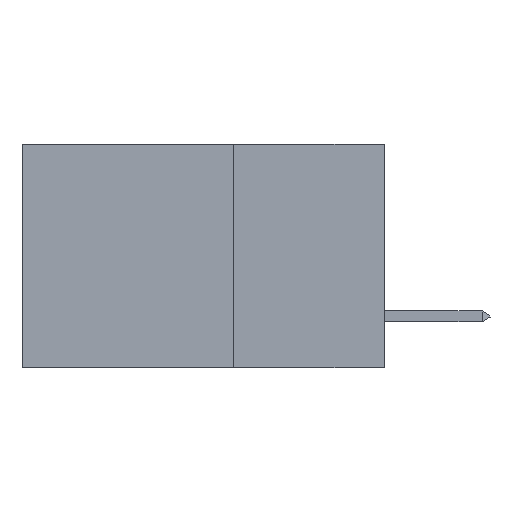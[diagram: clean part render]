
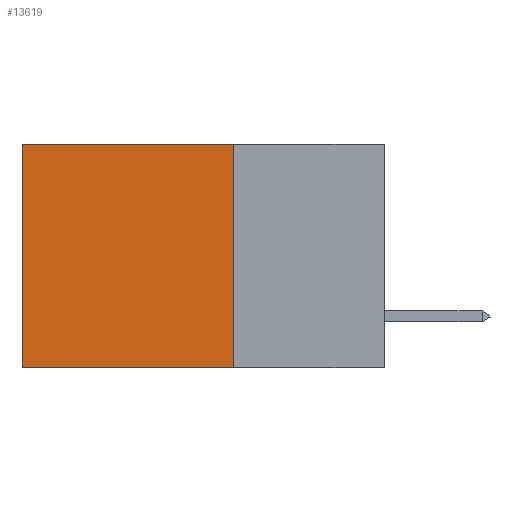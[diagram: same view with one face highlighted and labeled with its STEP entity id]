
A CAD part, left-side view. The second image highlights one B-rep face of the part: STEP entity #13619.
In plain terms, the highlighted planar face has unit normal (-1, 0, 0).
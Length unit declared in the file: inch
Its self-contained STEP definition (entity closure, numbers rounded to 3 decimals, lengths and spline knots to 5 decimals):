
#295 = EDGE_CURVE ( 'NONE', #6804, #10270, #2146, .T. ) ;
#1243 = CARTESIAN_POINT ( 'NONE',  ( 0.2875, 0.6, 0. ) ) ;
#1862 = CARTESIAN_POINT ( 'NONE',  ( 0.2875, 0.6, 0. ) ) ;
#2146 = LINE ( 'NONE', #15184, #16789 ) ;
#2931 = DIRECTION ( 'NONE',  ( 1., 0., 0. ) ) ;
#3605 = DIRECTION ( 'NONE',  ( 0., 0., -1. ) ) ;
#4009 = CARTESIAN_POINT ( 'NONE',  ( 0.2875, 0.25, 0. ) ) ;
#4480 = EDGE_CURVE ( 'NONE', #6804, #11323, #6038, .T. ) ;
#5873 = ORIENTED_EDGE ( 'NONE', *, *, #4480, .T. ) ;
#6038 = LINE ( 'NONE', #4009, #15990 ) ;
#6400 = FACE_OUTER_BOUND ( 'NONE', #13943, .T. ) ;
#6772 = ORIENTED_EDGE ( 'NONE', *, *, #13091, .T. ) ;
#6804 = VERTEX_POINT ( 'NONE', #10880 ) ;
#7690 = DIRECTION ( 'NONE',  ( 0., 1., 0. ) ) ;
#8319 = AXIS2_PLACEMENT_3D ( 'NONE', #9859, #2931, #12002 ) ;
#9859 = CARTESIAN_POINT ( 'NONE',  ( 0.2875, 0.25, 0. ) ) ;
#9945 = DIRECTION ( 'NONE',  ( 0., 1., 0. ) ) ;
#10129 = ORIENTED_EDGE ( 'NONE', *, *, #295, .F. ) ;
#10270 = VERTEX_POINT ( 'NONE', #15172 ) ;
#10651 = ORIENTED_EDGE ( 'NONE', *, *, #16809, .F. ) ;
#10689 = PLANE ( 'NONE',  #8319 ) ;
#10880 = CARTESIAN_POINT ( 'NONE',  ( 0.2875, 0.25, 0. ) ) ;
#11086 = CARTESIAN_POINT ( 'NONE',  ( 0.2875, 0.6, -0.37 ) ) ;
#11323 = VERTEX_POINT ( 'NONE', #1862 ) ;
#12002 = DIRECTION ( 'NONE',  ( 0., 0., -1. ) ) ;
#12082 = LINE ( 'NONE', #16307, #13721 ) ;
#12824 = DIRECTION ( 'NONE',  ( 0., 0., -1. ) ) ;
#13091 = EDGE_CURVE ( 'NONE', #11323, #14695, #14935, .T. ) ;
#13619 = ADVANCED_FACE ( 'NONE', ( #6400 ), #10689, .F. ) ;
#13721 = VECTOR ( 'NONE', #9945, 39.37008 ) ;
#13943 = EDGE_LOOP ( 'NONE', ( #6772, #10651, #10129, #5873 ) ) ;
#14695 = VERTEX_POINT ( 'NONE', #11086 ) ;
#14935 = LINE ( 'NONE', #1243, #15373 ) ;
#15172 = CARTESIAN_POINT ( 'NONE',  ( 0.2875, 0.25, -0.37 ) ) ;
#15184 = CARTESIAN_POINT ( 'NONE',  ( 0.2875, 0.25, 0. ) ) ;
#15373 = VECTOR ( 'NONE', #12824, 39.37008 ) ;
#15990 = VECTOR ( 'NONE', #7690, 39.37008 ) ;
#16307 = CARTESIAN_POINT ( 'NONE',  ( 0.2875, 0.25, -0.37 ) ) ;
#16789 = VECTOR ( 'NONE', #3605, 39.37008 ) ;
#16809 = EDGE_CURVE ( 'NONE', #10270, #14695, #12082, .T. ) ;
